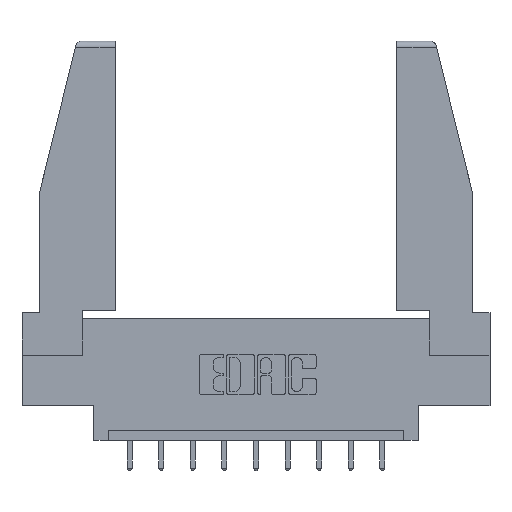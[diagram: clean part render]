
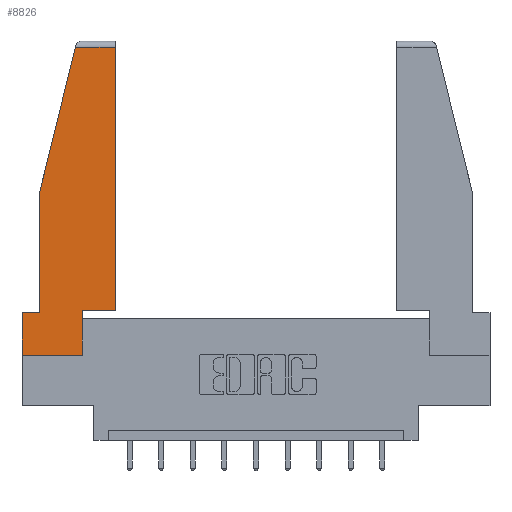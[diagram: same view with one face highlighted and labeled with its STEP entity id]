
A CAD part, top view. The second image highlights one B-rep face of the part: STEP entity #8826.
In plain terms, the highlighted planar face has unit normal (0, 0, 1).
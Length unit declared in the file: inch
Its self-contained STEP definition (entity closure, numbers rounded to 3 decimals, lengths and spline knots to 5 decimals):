
#250 = EDGE_CURVE ( 'NONE', #12511, #2654, #7324, .T. ) ;
#268 = VECTOR ( 'NONE', #2136, 39.37008 ) ;
#372 = VERTEX_POINT ( 'NONE', #9425 ) ;
#498 = EDGE_CURVE ( 'NONE', #9012, #4206, #3026, .T. ) ;
#578 = CARTESIAN_POINT ( 'NONE',  ( 0.461, 0.223, 0. ) ) ;
#631 = EDGE_CURVE ( 'NONE', #4206, #13376, #12034, .T. ) ;
#638 = DIRECTION ( 'NONE',  ( -1., 0., 0. ) ) ;
#1537 = ORIENTED_EDGE ( 'NONE', *, *, #250, .T. ) ;
#1556 = VERTEX_POINT ( 'NONE', #3654 ) ;
#1633 = CARTESIAN_POINT ( 'NONE',  ( 0.086, 0.8, 0. ) ) ;
#1794 = CARTESIAN_POINT ( 'NONE',  ( 0., 0., 0. ) ) ;
#1984 = ORIENTED_EDGE ( 'NONE', *, *, #2346, .T. ) ;
#2136 = DIRECTION ( 'NONE',  ( 0., 1., 0. ) ) ;
#2346 = EDGE_CURVE ( 'NONE', #372, #5088, #4494, .T. ) ;
#2654 = VERTEX_POINT ( 'NONE', #9086 ) ;
#3013 = LINE ( 'NONE', #11785, #12683 ) ;
#3026 = LINE ( 'NONE', #4353, #268 ) ;
#3526 = DIRECTION ( 'NONE',  ( -0.239, -0.971, 0. ) ) ;
#3654 = CARTESIAN_POINT ( 'NONE',  ( 0.086, 0.8, 0. ) ) ;
#3722 = CARTESIAN_POINT ( 'NONE',  ( 0.297, 0., 0. ) ) ;
#4151 = CARTESIAN_POINT ( 'NONE',  ( 0., 0.21, 0. ) ) ;
#4206 = VERTEX_POINT ( 'NONE', #4877 ) ;
#4306 = EDGE_CURVE ( 'NONE', #10068, #9012, #11605, .T. ) ;
#4353 = CARTESIAN_POINT ( 'NONE',  ( 0.461, 0.223, 0. ) ) ;
#4494 = LINE ( 'NONE', #4151, #6969 ) ;
#4536 = VECTOR ( 'NONE', #8172, 39.37008 ) ;
#4858 = VECTOR ( 'NONE', #638, 39.37008 ) ;
#4877 = CARTESIAN_POINT ( 'NONE',  ( 0.461, 1.52, 0. ) ) ;
#5084 = ORIENTED_EDGE ( 'NONE', *, *, #631, .T. ) ;
#5088 = VERTEX_POINT ( 'NONE', #13081 ) ;
#5446 = ORIENTED_EDGE ( 'NONE', *, *, #9001, .T. ) ;
#6044 = PLANE ( 'NONE',  #10500 ) ;
#6177 = DIRECTION ( 'NONE',  ( -1., 0., 0. ) ) ;
#6317 = CARTESIAN_POINT ( 'NONE',  ( 0.297, 0.223, 0. ) ) ;
#6416 = ORIENTED_EDGE ( 'NONE', *, *, #7111, .T. ) ;
#6503 = DIRECTION ( 'NONE',  ( 0., -1., 0. ) ) ;
#6830 = ORIENTED_EDGE ( 'NONE', *, *, #4306, .T. ) ;
#6870 = CARTESIAN_POINT ( 'NONE',  ( 0., 0., 0. ) ) ;
#6969 = VECTOR ( 'NONE', #6177, 39.37008 ) ;
#7087 = FACE_OUTER_BOUND ( 'NONE', #13325, .T. ) ;
#7105 = DIRECTION ( 'NONE',  ( 0., 0., 1. ) ) ;
#7111 = EDGE_CURVE ( 'NONE', #13376, #1556, #3013, .T. ) ;
#7189 = VECTOR ( 'NONE', #6503, 39.37008 ) ;
#7324 = LINE ( 'NONE', #1794, #4536 ) ;
#7901 = ORIENTED_EDGE ( 'NONE', *, *, #12933, .T. ) ;
#8172 = DIRECTION ( 'NONE',  ( 1., 0., 0. ) ) ;
#8327 = LINE ( 'NONE', #1633, #7189 ) ;
#8383 = LINE ( 'NONE', #3722, #9824 ) ;
#8826 = ADVANCED_FACE ( 'NONE', ( #7087 ), #6044, .T. ) ;
#8839 = VECTOR ( 'NONE', #12136, 39.37008 ) ;
#9001 = EDGE_CURVE ( 'NONE', #2654, #10068, #8383, .T. ) ;
#9012 = VERTEX_POINT ( 'NONE', #578 ) ;
#9080 = CARTESIAN_POINT ( 'NONE',  ( 0.2636, 1.52, 0. ) ) ;
#9086 = CARTESIAN_POINT ( 'NONE',  ( 0.297, 0., 0. ) ) ;
#9330 = ORIENTED_EDGE ( 'NONE', *, *, #498, .T. ) ;
#9425 = CARTESIAN_POINT ( 'NONE',  ( 0.086, 0.21, 0. ) ) ;
#9824 = VECTOR ( 'NONE', #13070, 39.37008 ) ;
#9890 = EDGE_CURVE ( 'NONE', #5088, #12511, #10780, .T. ) ;
#9905 = CARTESIAN_POINT ( 'NONE',  ( 0., 1.52, 0. ) ) ;
#10068 = VERTEX_POINT ( 'NONE', #6317 ) ;
#10500 = AXIS2_PLACEMENT_3D ( 'NONE', #13356, #7105, #11258 ) ;
#10613 = VECTOR ( 'NONE', #10694, 39.37008 ) ;
#10649 = CARTESIAN_POINT ( 'NONE',  ( 0.297, 0.223, 0. ) ) ;
#10694 = DIRECTION ( 'NONE',  ( 1., 0., 0. ) ) ;
#10780 = LINE ( 'NONE', #13362, #8839 ) ;
#10829 = ORIENTED_EDGE ( 'NONE', *, *, #9890, .T. ) ;
#11258 = DIRECTION ( 'NONE',  ( 1., 0., 0. ) ) ;
#11605 = LINE ( 'NONE', #10649, #10613 ) ;
#11785 = CARTESIAN_POINT ( 'NONE',  ( 0.271, 1.55, 0. ) ) ;
#12034 = LINE ( 'NONE', #9905, #4858 ) ;
#12136 = DIRECTION ( 'NONE',  ( 0., -1., 0. ) ) ;
#12511 = VERTEX_POINT ( 'NONE', #6870 ) ;
#12683 = VECTOR ( 'NONE', #3526, 39.37008 ) ;
#12933 = EDGE_CURVE ( 'NONE', #1556, #372, #8327, .T. ) ;
#13070 = DIRECTION ( 'NONE',  ( 0., 1., 0. ) ) ;
#13081 = CARTESIAN_POINT ( 'NONE',  ( 0., 0.21, 0. ) ) ;
#13325 = EDGE_LOOP ( 'NONE', ( #9330, #5084, #6416, #7901, #1984, #10829, #1537, #5446, #6830 ) ) ;
#13356 = CARTESIAN_POINT ( 'NONE',  ( 0., 0., 0. ) ) ;
#13362 = CARTESIAN_POINT ( 'NONE',  ( 0., 0.21, 0. ) ) ;
#13376 = VERTEX_POINT ( 'NONE', #9080 ) ;
